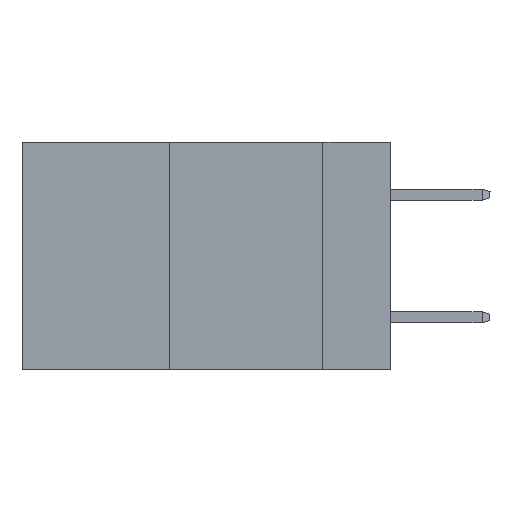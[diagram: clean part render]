
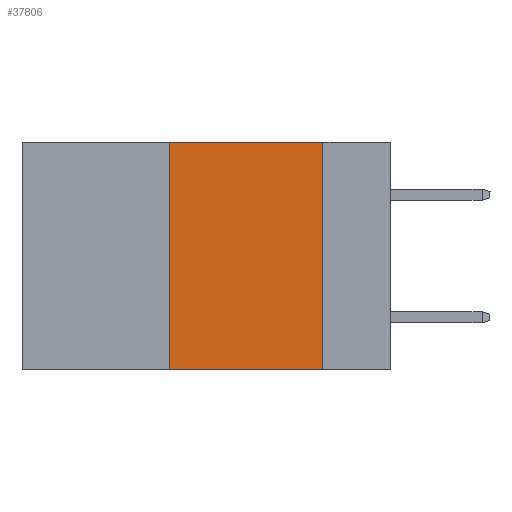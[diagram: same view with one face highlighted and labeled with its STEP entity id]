
A CAD part, left-side view. The second image highlights one B-rep face of the part: STEP entity #37806.
In plain terms, the highlighted planar face has unit normal (-1, 0, 0).
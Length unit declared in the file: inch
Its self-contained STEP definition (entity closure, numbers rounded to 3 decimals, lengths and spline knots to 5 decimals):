
#1708 = VERTEX_POINT ( 'NONE', #28369 ) ;
#2810 = VECTOR ( 'NONE', #4975, 39.37008 ) ;
#3772 = CARTESIAN_POINT ( 'NONE',  ( 0., 0.36, 0. ) ) ;
#4975 = DIRECTION ( 'NONE',  ( 0., -1., 0. ) ) ;
#5478 = EDGE_CURVE ( 'NONE', #24671, #1708, #39184, .T. ) ;
#6348 = EDGE_CURVE ( 'NONE', #15123, #24671, #14124, .T. ) ;
#6748 = VERTEX_POINT ( 'NONE', #25857 ) ;
#6966 = FACE_OUTER_BOUND ( 'NONE', #25126, .T. ) ;
#9061 = DIRECTION ( 'NONE',  ( 1., 0., 0. ) ) ;
#9472 = CARTESIAN_POINT ( 'NONE',  ( 0., 0.36, 0. ) ) ;
#12482 = EDGE_CURVE ( 'NONE', #1708, #6748, #19759, .T. ) ;
#13050 = VECTOR ( 'NONE', #23172, 39.37008 ) ;
#14124 = LINE ( 'NONE', #9472, #13050 ) ;
#15123 = VERTEX_POINT ( 'NONE', #43461 ) ;
#16948 = AXIS2_PLACEMENT_3D ( 'NONE', #29673, #9061, #33052 ) ;
#19759 = LINE ( 'NONE', #25994, #36743 ) ;
#20670 = CARTESIAN_POINT ( 'NONE',  ( 0., 0.6, -0.37 ) ) ;
#22190 = CARTESIAN_POINT ( 'NONE',  ( 0., 0.6, 0. ) ) ;
#22554 = DIRECTION ( 'NONE',  ( 0., 0., -1. ) ) ;
#22770 = PLANE ( 'NONE',  #16948 ) ;
#23172 = DIRECTION ( 'NONE',  ( 0., 0., 1. ) ) ;
#24671 = VERTEX_POINT ( 'NONE', #3772 ) ;
#25055 = ORIENTED_EDGE ( 'NONE', *, *, #12482, .F. ) ;
#25126 = EDGE_LOOP ( 'NONE', ( #25055, #25780, #26517, #26777 ) ) ;
#25780 = ORIENTED_EDGE ( 'NONE', *, *, #5478, .F. ) ;
#25857 = CARTESIAN_POINT ( 'NONE',  ( 0., 0.11, -0.37 ) ) ;
#25994 = CARTESIAN_POINT ( 'NONE',  ( 0., 0.11, 0. ) ) ;
#26517 = ORIENTED_EDGE ( 'NONE', *, *, #6348, .F. ) ;
#26777 = ORIENTED_EDGE ( 'NONE', *, *, #39213, .T. ) ;
#28369 = CARTESIAN_POINT ( 'NONE',  ( 0., 0.11, 0. ) ) ;
#29673 = CARTESIAN_POINT ( 'NONE',  ( 0., 0.6, 0. ) ) ;
#30022 = LINE ( 'NONE', #20670, #37837 ) ;
#33052 = DIRECTION ( 'NONE',  ( 0., 0., -1. ) ) ;
#36743 = VECTOR ( 'NONE', #22554, 39.37008 ) ;
#37708 = DIRECTION ( 'NONE',  ( 0., -1., 0. ) ) ;
#37806 = ADVANCED_FACE ( 'NONE', ( #6966 ), #22770, .F. ) ;
#37837 = VECTOR ( 'NONE', #37708, 39.37008 ) ;
#39184 = LINE ( 'NONE', #22190, #2810 ) ;
#39213 = EDGE_CURVE ( 'NONE', #15123, #6748, #30022, .T. ) ;
#43461 = CARTESIAN_POINT ( 'NONE',  ( 0., 0.36, -0.37 ) ) ;
